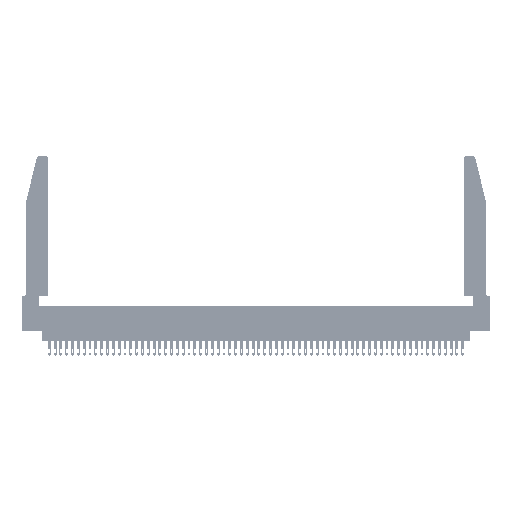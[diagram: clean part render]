
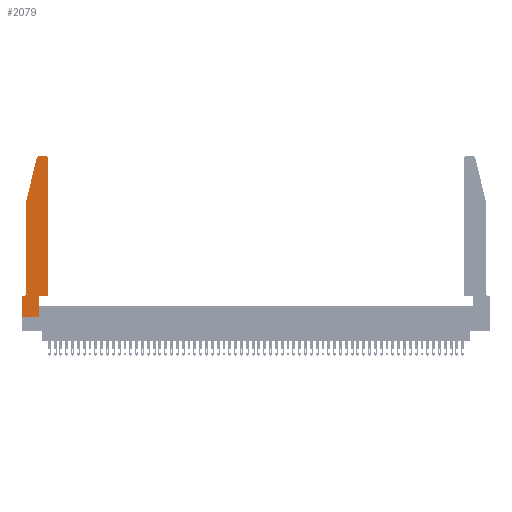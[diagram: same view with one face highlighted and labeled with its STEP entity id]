
A CAD part, top view. The second image highlights one B-rep face of the part: STEP entity #2079.
In plain terms, the highlighted planar face has unit normal (0, 0, 1).
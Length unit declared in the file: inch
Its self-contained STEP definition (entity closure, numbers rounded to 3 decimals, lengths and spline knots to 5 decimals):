
#457 = CIRCLE ( 'NONE', #3087, 0.03 ) ;
#1186 = ORIENTED_EDGE ( 'NONE', *, *, #51219, .T. ) ;
#2079 = ADVANCED_FACE ( 'NONE', ( #56072 ), #6114, .T. ) ;
#2896 = AXIS2_PLACEMENT_3D ( 'NONE', #7523, #43207, #29875 ) ;
#3087 = AXIS2_PLACEMENT_3D ( 'NONE', #42717, #20704, #29585 ) ;
#3301 = VERTEX_POINT ( 'NONE', #19301 ) ;
#3427 = CARTESIAN_POINT ( 'NONE',  ( 0.2865, 0.35, 0.37 ) ) ;
#3695 = VECTOR ( 'NONE', #7323, 39.37008 ) ;
#5860 = DIRECTION ( 'NONE',  ( -1., 0., 0. ) ) ;
#6114 = PLANE ( 'NONE',  #27600 ) ;
#6479 = VECTOR ( 'NONE', #56898, 39.37008 ) ;
#7323 = DIRECTION ( 'NONE',  ( 0., 1., 0. ) ) ;
#7388 = AXIS2_PLACEMENT_3D ( 'NONE', #31764, #31570, #9810 ) ;
#7406 = CARTESIAN_POINT ( 'NONE',  ( 0.0055, 0.35, 0.37 ) ) ;
#7512 = EDGE_LOOP ( 'NONE', ( #45089, #38856, #50150, #57221, #17119, #19559, #26458, #39389, #8505, #27244, #1186, #22270 ) ) ;
#7523 = CARTESIAN_POINT ( 'NONE',  ( 0.0055, 0.42, 0.37 ) ) ;
#8309 = DIRECTION ( 'NONE',  ( -0.239, -0.971, 0. ) ) ;
#8505 = ORIENTED_EDGE ( 'NONE', *, *, #16374, .T. ) ;
#8539 = DIRECTION ( 'NONE',  ( 1., 0., 0. ) ) ;
#9217 = DIRECTION ( 'NONE',  ( 1., 0., 0. ) ) ;
#9704 = DIRECTION ( 'NONE',  ( 0., -1., 0. ) ) ;
#9810 = DIRECTION ( 'NONE',  ( 1., 0., 0. ) ) ;
#11867 = CIRCLE ( 'NONE', #2896, 0.07 ) ;
#12264 = VECTOR ( 'NONE', #8309, 39.37008 ) ;
#12955 = LINE ( 'NONE', #53276, #48191 ) ;
#13908 = VECTOR ( 'NONE', #9704, 39.37008 ) ;
#14167 = LINE ( 'NONE', #28068, #43861 ) ;
#14592 = DIRECTION ( 'NONE',  ( 1., 0., 0. ) ) ;
#14717 = LINE ( 'NONE', #31056, #17471 ) ;
#15740 = LINE ( 'NONE', #19005, #40635 ) ;
#16374 = EDGE_CURVE ( 'NONE', #32645, #37851, #45893, .T. ) ;
#16627 = EDGE_CURVE ( 'NONE', #24339, #49553, #47224, .T. ) ;
#17119 = ORIENTED_EDGE ( 'NONE', *, *, #26981, .T. ) ;
#17471 = VECTOR ( 'NONE', #8539, 39.37008 ) ;
#18714 = LINE ( 'NONE', #27232, #13908 ) ;
#19005 = CARTESIAN_POINT ( 'NONE',  ( 0.4505, 0.35, 0.37 ) ) ;
#19301 = CARTESIAN_POINT ( 'NONE',  ( 0.0755, 2., 0.37 ) ) ;
#19559 = ORIENTED_EDGE ( 'NONE', *, *, #25081, .T. ) ;
#20704 = DIRECTION ( 'NONE',  ( 0., 0., 1. ) ) ;
#21192 = LINE ( 'NONE', #52360, #12264 ) ;
#22270 = ORIENTED_EDGE ( 'NONE', *, *, #16627, .T. ) ;
#22906 = EDGE_CURVE ( 'NONE', #45525, #32645, #12955, .T. ) ;
#23228 = CARTESIAN_POINT ( 'NONE',  ( 0.2605, 2.75, 0.37 ) ) ;
#24001 = CARTESIAN_POINT ( 'NONE',  ( 0.2865, 0., 0.37 ) ) ;
#24339 = VERTEX_POINT ( 'NONE', #53742 ) ;
#24409 = LINE ( 'NONE', #55953, #6479 ) ;
#25081 = EDGE_CURVE ( 'NONE', #32744, #27693, #14167, .T. ) ;
#25891 = EDGE_CURVE ( 'NONE', #3301, #56991, #18714, .T. ) ;
#26458 = ORIENTED_EDGE ( 'NONE', *, *, #32749, .T. ) ;
#26981 = EDGE_CURVE ( 'NONE', #56991, #32744, #11867, .T. ) ;
#27232 = CARTESIAN_POINT ( 'NONE',  ( 0.0755, 2., 0.37 ) ) ;
#27244 = ORIENTED_EDGE ( 'NONE', *, *, #49042, .T. ) ;
#27600 = AXIS2_PLACEMENT_3D ( 'NONE', #28469, #37329, #14592 ) ;
#27693 = VERTEX_POINT ( 'NONE', #38304 ) ;
#27873 = DIRECTION ( 'NONE',  ( 0., 1., 0. ) ) ;
#28068 = CARTESIAN_POINT ( 'NONE',  ( 0.0755, 0.35, 0.37 ) ) ;
#28469 = CARTESIAN_POINT ( 'NONE',  ( 0., 0.35, 0.37 ) ) ;
#29200 = CARTESIAN_POINT ( 'NONE',  ( 0.284, 2.75, 0.37 ) ) ;
#29585 = DIRECTION ( 'NONE',  ( 1., 0., 0. ) ) ;
#29875 = DIRECTION ( 'NONE',  ( -1., 0., 0. ) ) ;
#30077 = EDGE_CURVE ( 'NONE', #40073, #3301, #21192, .T. ) ;
#30319 = CARTESIAN_POINT ( 'NONE',  ( 0.4505, 0.35, 0.37 ) ) ;
#30391 = CARTESIAN_POINT ( 'NONE',  ( 0.2865, 0.35, 0.37 ) ) ;
#30910 = CARTESIAN_POINT ( 'NONE',  ( 0.25487, 2.72718, 0.37 ) ) ;
#31056 = CARTESIAN_POINT ( 'NONE',  ( 0.4505, 0.35, 0.37 ) ) ;
#31212 = EDGE_CURVE ( 'NONE', #51375, #40073, #457, .T. ) ;
#31570 = DIRECTION ( 'NONE',  ( 0., 0., 1. ) ) ;
#31764 = CARTESIAN_POINT ( 'NONE',  ( 0.4205, 2.72, 0.37 ) ) ;
#32645 = VERTEX_POINT ( 'NONE', #24001 ) ;
#32744 = VERTEX_POINT ( 'NONE', #7406 ) ;
#32749 = EDGE_CURVE ( 'NONE', #27693, #45525, #24409, .T. ) ;
#34351 = EDGE_CURVE ( 'NONE', #49553, #51375, #40111, .T. ) ;
#37329 = DIRECTION ( 'NONE',  ( 0., 0., 1. ) ) ;
#37851 = VERTEX_POINT ( 'NONE', #30391 ) ;
#38304 = CARTESIAN_POINT ( 'NONE',  ( 0., 0.35, 0.37 ) ) ;
#38856 = ORIENTED_EDGE ( 'NONE', *, *, #31212, .T. ) ;
#38940 = CARTESIAN_POINT ( 'NONE',  ( 0.4205, 2.75, 0.37 ) ) ;
#39389 = ORIENTED_EDGE ( 'NONE', *, *, #22906, .T. ) ;
#40073 = VERTEX_POINT ( 'NONE', #30910 ) ;
#40111 = LINE ( 'NONE', #23228, #51908 ) ;
#40635 = VECTOR ( 'NONE', #27873, 39.37008 ) ;
#42717 = CARTESIAN_POINT ( 'NONE',  ( 0.284, 2.72, 0.37 ) ) ;
#43207 = DIRECTION ( 'NONE',  ( 0., 0., -1. ) ) ;
#43861 = VECTOR ( 'NONE', #49572, 39.37008 ) ;
#45089 = ORIENTED_EDGE ( 'NONE', *, *, #34351, .T. ) ;
#45525 = VERTEX_POINT ( 'NONE', #57235 ) ;
#45893 = LINE ( 'NONE', #3427, #3695 ) ;
#47224 = CIRCLE ( 'NONE', #7388, 0.03 ) ;
#47933 = CARTESIAN_POINT ( 'NONE',  ( 0.0755, 0.42, 0.37 ) ) ;
#48191 = VECTOR ( 'NONE', #9217, 39.37008 ) ;
#49042 = EDGE_CURVE ( 'NONE', #37851, #57231, #14717, .T. ) ;
#49553 = VERTEX_POINT ( 'NONE', #38940 ) ;
#49572 = DIRECTION ( 'NONE',  ( -1., 0., 0. ) ) ;
#50150 = ORIENTED_EDGE ( 'NONE', *, *, #30077, .T. ) ;
#51219 = EDGE_CURVE ( 'NONE', #57231, #24339, #15740, .T. ) ;
#51375 = VERTEX_POINT ( 'NONE', #29200 ) ;
#51908 = VECTOR ( 'NONE', #5860, 39.37008 ) ;
#52360 = CARTESIAN_POINT ( 'NONE',  ( 0.0755, 2., 0.37 ) ) ;
#53276 = CARTESIAN_POINT ( 'NONE',  ( 0., 0., 0.37 ) ) ;
#53742 = CARTESIAN_POINT ( 'NONE',  ( 0.4505, 2.72, 0.37 ) ) ;
#55953 = CARTESIAN_POINT ( 'NONE',  ( 0., 0., 0.37 ) ) ;
#56072 = FACE_OUTER_BOUND ( 'NONE', #7512, .T. ) ;
#56898 = DIRECTION ( 'NONE',  ( 0., -1., 0. ) ) ;
#56991 = VERTEX_POINT ( 'NONE', #47933 ) ;
#57221 = ORIENTED_EDGE ( 'NONE', *, *, #25891, .T. ) ;
#57231 = VERTEX_POINT ( 'NONE', #30319 ) ;
#57235 = CARTESIAN_POINT ( 'NONE',  ( 0., 0., 0.37 ) ) ;
